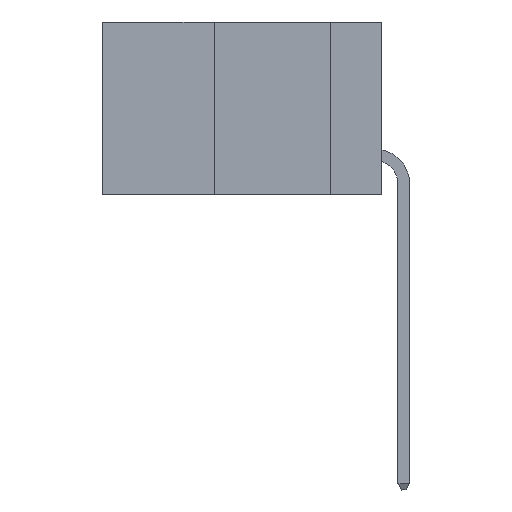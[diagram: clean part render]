
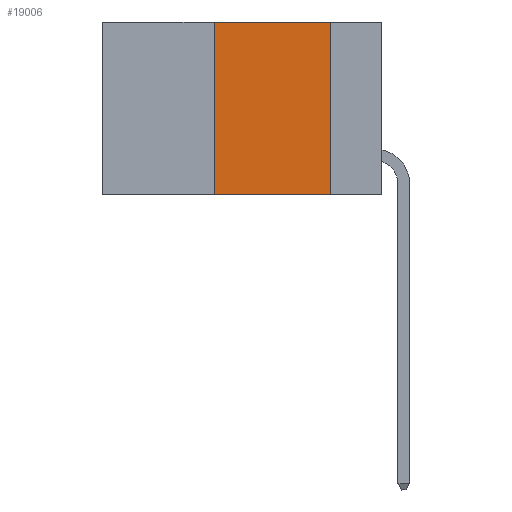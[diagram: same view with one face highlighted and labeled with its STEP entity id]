
A CAD part, left-side view. The second image highlights one B-rep face of the part: STEP entity #19006.
In plain terms, the highlighted planar face has unit normal (-1, 0, 0).
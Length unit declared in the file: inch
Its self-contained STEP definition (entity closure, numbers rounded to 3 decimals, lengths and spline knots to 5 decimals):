
#790 = VECTOR ( 'NONE', #27994, 39.37008 ) ;
#1065 = DIRECTION ( 'NONE',  ( 0., -1., 0. ) ) ;
#2436 = AXIS2_PLACEMENT_3D ( 'NONE', #20314, #38000, #13856 ) ;
#3471 = CARTESIAN_POINT ( 'NONE',  ( 0., 0.11, 0. ) ) ;
#4010 = CARTESIAN_POINT ( 'NONE',  ( 0., 0.11, 0. ) ) ;
#4068 = EDGE_CURVE ( 'NONE', #17455, #13357, #37569, .T. ) ;
#5638 = DIRECTION ( 'NONE',  ( 0., -1., 0. ) ) ;
#7661 = CARTESIAN_POINT ( 'NONE',  ( 0., 0.6, 0. ) ) ;
#9243 = ORIENTED_EDGE ( 'NONE', *, *, #26298, .F. ) ;
#9722 = EDGE_CURVE ( 'NONE', #12583, #22450, #25681, .T. ) ;
#12583 = VERTEX_POINT ( 'NONE', #45205 ) ;
#13357 = VERTEX_POINT ( 'NONE', #41833 ) ;
#13409 = PLANE ( 'NONE',  #2436 ) ;
#13856 = DIRECTION ( 'NONE',  ( 0., 0., -1. ) ) ;
#17455 = VERTEX_POINT ( 'NONE', #24496 ) ;
#19006 = ADVANCED_FACE ( 'NONE', ( #36522 ), #13409, .F. ) ;
#19362 = LINE ( 'NONE', #25711, #28087 ) ;
#20314 = CARTESIAN_POINT ( 'NONE',  ( 0., 0.6, 0. ) ) ;
#22450 = VERTEX_POINT ( 'NONE', #4010 ) ;
#24496 = CARTESIAN_POINT ( 'NONE',  ( 0., 0.36, -0.37 ) ) ;
#25559 = DIRECTION ( 'NONE',  ( 0., 0., 1. ) ) ;
#25681 = LINE ( 'NONE', #7661, #36147 ) ;
#25711 = CARTESIAN_POINT ( 'NONE',  ( 0., 0.36, 0. ) ) ;
#26298 = EDGE_CURVE ( 'NONE', #17455, #12583, #19362, .T. ) ;
#27994 = DIRECTION ( 'NONE',  ( 0., 0., -1. ) ) ;
#28087 = VECTOR ( 'NONE', #25559, 39.37008 ) ;
#31551 = EDGE_CURVE ( 'NONE', #22450, #13357, #38152, .T. ) ;
#34249 = VECTOR ( 'NONE', #5638, 39.37008 ) ;
#35620 = ORIENTED_EDGE ( 'NONE', *, *, #31551, .F. ) ;
#35754 = EDGE_LOOP ( 'NONE', ( #35620, #44335, #9243, #43054 ) ) ;
#36147 = VECTOR ( 'NONE', #1065, 39.37008 ) ;
#36522 = FACE_OUTER_BOUND ( 'NONE', #35754, .T. ) ;
#36808 = CARTESIAN_POINT ( 'NONE',  ( 0., 0.6, -0.37 ) ) ;
#37569 = LINE ( 'NONE', #36808, #34249 ) ;
#38000 = DIRECTION ( 'NONE',  ( 1., 0., 0. ) ) ;
#38152 = LINE ( 'NONE', #3471, #790 ) ;
#41833 = CARTESIAN_POINT ( 'NONE',  ( 0., 0.11, -0.37 ) ) ;
#43054 = ORIENTED_EDGE ( 'NONE', *, *, #4068, .T. ) ;
#44335 = ORIENTED_EDGE ( 'NONE', *, *, #9722, .F. ) ;
#45205 = CARTESIAN_POINT ( 'NONE',  ( 0., 0.36, 0. ) ) ;
